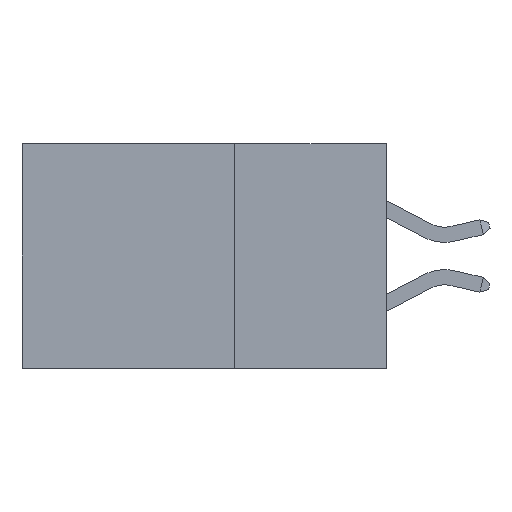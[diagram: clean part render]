
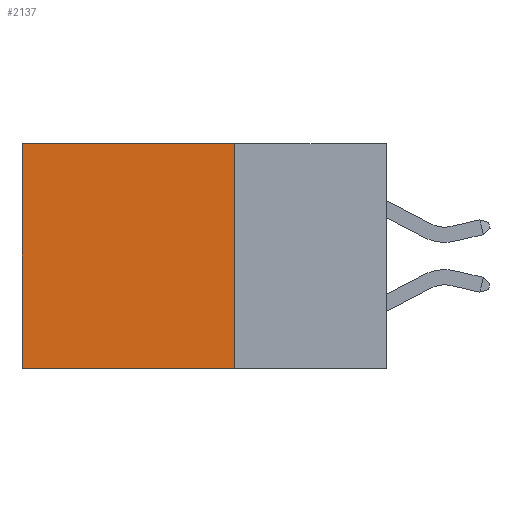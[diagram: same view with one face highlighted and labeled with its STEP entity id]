
A CAD part, left-side view. The second image highlights one B-rep face of the part: STEP entity #2137.
In plain terms, the highlighted planar face has unit normal (-1, 0, 0).
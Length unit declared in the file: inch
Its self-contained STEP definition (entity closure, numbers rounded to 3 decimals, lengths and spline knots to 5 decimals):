
#46 = EDGE_CURVE ( 'NONE', #7533, #3275, #2994, .T. ) ;
#337 = LINE ( 'NONE', #7328, #9317 ) ;
#1076 = ORIENTED_EDGE ( 'NONE', *, *, #7996, .F. ) ;
#1172 = VERTEX_POINT ( 'NONE', #7970 ) ;
#1212 = EDGE_LOOP ( 'NONE', ( #8005, #1076, #5790, #6723 ) ) ;
#1588 = CARTESIAN_POINT ( 'NONE',  ( 0.298, 0.25, 0. ) ) ;
#1641 = AXIS2_PLACEMENT_3D ( 'NONE', #4296, #5777, #6528 ) ;
#1914 = DIRECTION ( 'NONE',  ( 0., 1., 0. ) ) ;
#2137 = ADVANCED_FACE ( 'NONE', ( #5377 ), #8819, .F. ) ;
#2161 = CARTESIAN_POINT ( 'NONE',  ( 0.298, 0.6, 0. ) ) ;
#2552 = LINE ( 'NONE', #3359, #8075 ) ;
#2994 = LINE ( 'NONE', #5674, #5866 ) ;
#3151 = EDGE_CURVE ( 'NONE', #3275, #1172, #337, .T. ) ;
#3275 = VERTEX_POINT ( 'NONE', #2161 ) ;
#3359 = CARTESIAN_POINT ( 'NONE',  ( 0.298, 0.25, 0. ) ) ;
#4250 = CARTESIAN_POINT ( 'NONE',  ( 0.298, 0.25, -0.37 ) ) ;
#4296 = CARTESIAN_POINT ( 'NONE',  ( 0.298, 0.25, 0. ) ) ;
#5073 = CARTESIAN_POINT ( 'NONE',  ( 0.298, 0.25, -0.37 ) ) ;
#5116 = VERTEX_POINT ( 'NONE', #5073 ) ;
#5377 = FACE_OUTER_BOUND ( 'NONE', #1212, .T. ) ;
#5547 = DIRECTION ( 'NONE',  ( 0., 0., -1. ) ) ;
#5674 = CARTESIAN_POINT ( 'NONE',  ( 0.298, 0.25, 0. ) ) ;
#5768 = LINE ( 'NONE', #4250, #6800 ) ;
#5777 = DIRECTION ( 'NONE',  ( 1., 0., 0. ) ) ;
#5790 = ORIENTED_EDGE ( 'NONE', *, *, #7257, .F. ) ;
#5866 = VECTOR ( 'NONE', #1914, 39.37008 ) ;
#6528 = DIRECTION ( 'NONE',  ( 0., 0., -1. ) ) ;
#6621 = DIRECTION ( 'NONE',  ( 0., 0., -1. ) ) ;
#6723 = ORIENTED_EDGE ( 'NONE', *, *, #46, .T. ) ;
#6800 = VECTOR ( 'NONE', #9377, 39.37008 ) ;
#7257 = EDGE_CURVE ( 'NONE', #7533, #5116, #2552, .T. ) ;
#7328 = CARTESIAN_POINT ( 'NONE',  ( 0.298, 0.6, 0. ) ) ;
#7533 = VERTEX_POINT ( 'NONE', #1588 ) ;
#7970 = CARTESIAN_POINT ( 'NONE',  ( 0.298, 0.6, -0.37 ) ) ;
#7996 = EDGE_CURVE ( 'NONE', #5116, #1172, #5768, .T. ) ;
#8005 = ORIENTED_EDGE ( 'NONE', *, *, #3151, .T. ) ;
#8075 = VECTOR ( 'NONE', #5547, 39.37008 ) ;
#8819 = PLANE ( 'NONE',  #1641 ) ;
#9317 = VECTOR ( 'NONE', #6621, 39.37008 ) ;
#9377 = DIRECTION ( 'NONE',  ( 0., 1., 0. ) ) ;
